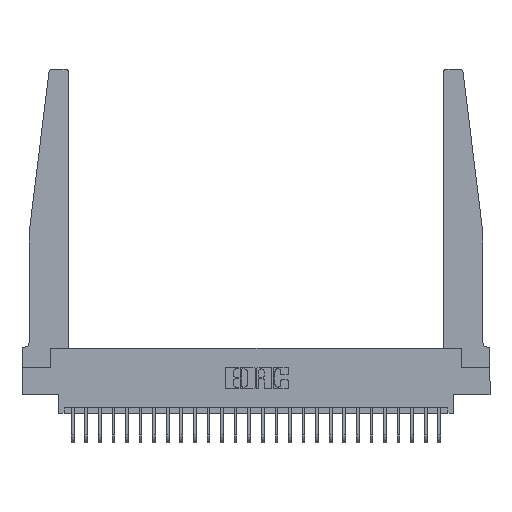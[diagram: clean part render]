
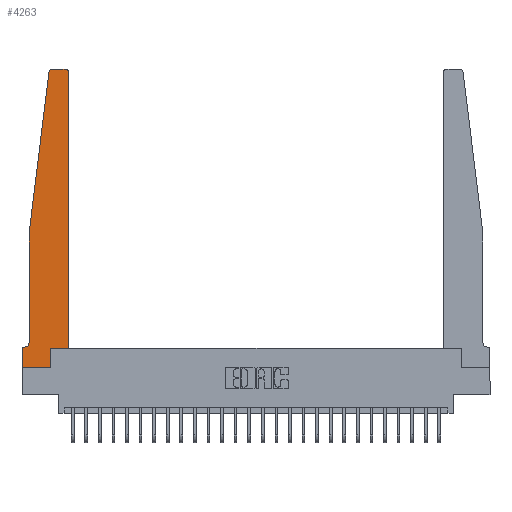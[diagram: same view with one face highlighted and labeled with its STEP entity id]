
A CAD part, top view. The second image highlights one B-rep face of the part: STEP entity #4263.
In plain terms, the highlighted planar face has unit normal (0, 0, 1).
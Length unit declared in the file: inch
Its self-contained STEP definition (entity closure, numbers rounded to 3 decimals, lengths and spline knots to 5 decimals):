
#93 = CARTESIAN_POINT ( 'NONE',  ( 0.425, 0.18, 0.37 ) ) ;
#144 = CARTESIAN_POINT ( 'NONE',  ( 0.015, 0.1875, 0.37 ) ) ;
#381 = DIRECTION ( 'NONE',  ( 1., 0., 0. ) ) ;
#610 = VECTOR ( 'NONE', #15739, 39.37008 ) ;
#1240 = AXIS2_PLACEMENT_3D ( 'NONE', #2203, #24949, #12525 ) ;
#1258 = CARTESIAN_POINT ( 'NONE',  ( 0.065, 0.1875, 0.37 ) ) ;
#2203 = CARTESIAN_POINT ( 'NONE',  ( 0.27653, 2.72, 0.37 ) ) ;
#2402 = CARTESIAN_POINT ( 'NONE',  ( 0.425, 0.18, 0.37 ) ) ;
#2494 = CARTESIAN_POINT ( 'NONE',  ( 0.2605, 0.18, 0.37 ) ) ;
#3144 = LINE ( 'NONE', #6841, #13518 ) ;
#3421 = ORIENTED_EDGE ( 'NONE', *, *, #20237, .T. ) ;
#3895 = LINE ( 'NONE', #1258, #610 ) ;
#4263 = ADVANCED_FACE ( 'NONE', ( #12003 ), #23340, .T. ) ;
#4941 = EDGE_CURVE ( 'NONE', #6797, #12315, #3895, .T. ) ;
#4987 = ORIENTED_EDGE ( 'NONE', *, *, #25589, .T. ) ;
#5059 = VERTEX_POINT ( 'NONE', #24735 ) ;
#5193 = CARTESIAN_POINT ( 'NONE',  ( 0.015, 0.2375, 0.37 ) ) ;
#5317 = EDGE_CURVE ( 'NONE', #20137, #15639, #16527, .T. ) ;
#5744 = CARTESIAN_POINT ( 'NONE',  ( 0., 0., 0.37 ) ) ;
#6098 = ORIENTED_EDGE ( 'NONE', *, *, #21970, .T. ) ;
#6454 = LINE ( 'NONE', #19128, #8363 ) ;
#6511 = LINE ( 'NONE', #9310, #22659 ) ;
#6797 = VERTEX_POINT ( 'NONE', #144 ) ;
#6841 = CARTESIAN_POINT ( 'NONE',  ( 0.25, 2.75, 0.37 ) ) ;
#7742 = EDGE_CURVE ( 'NONE', #5059, #6797, #14468, .T. ) ;
#7963 = ORIENTED_EDGE ( 'NONE', *, *, #19865, .T. ) ;
#8076 = DIRECTION ( 'NONE',  ( 1., 0., 0. ) ) ;
#8299 = CARTESIAN_POINT ( 'NONE',  ( 0.27653, 2.75, 0.37 ) ) ;
#8310 = AXIS2_PLACEMENT_3D ( 'NONE', #5193, #21519, #15535 ) ;
#8363 = VECTOR ( 'NONE', #10907, 39.37008 ) ;
#8761 = AXIS2_PLACEMENT_3D ( 'NONE', #12805, #14875, #381 ) ;
#8945 = EDGE_CURVE ( 'NONE', #13265, #20823, #6454, .T. ) ;
#9310 = CARTESIAN_POINT ( 'NONE',  ( 0., 0., 0.37 ) ) ;
#9668 = VERTEX_POINT ( 'NONE', #93 ) ;
#9821 = ORIENTED_EDGE ( 'NONE', *, *, #10875, .T. ) ;
#10350 = VECTOR ( 'NONE', #23063, 39.37008 ) ;
#10642 = CARTESIAN_POINT ( 'NONE',  ( 0.065, 1.25, 0.37 ) ) ;
#10706 = VERTEX_POINT ( 'NONE', #22304 ) ;
#10799 = VECTOR ( 'NONE', #16868, 39.37008 ) ;
#10838 = DIRECTION ( 'NONE',  ( 1., 0., 0. ) ) ;
#10875 = EDGE_CURVE ( 'NONE', #20823, #5059, #24450, .T. ) ;
#10907 = DIRECTION ( 'NONE',  ( -0.122, -0.992, 0. ) ) ;
#12003 = FACE_OUTER_BOUND ( 'NONE', #17654, .T. ) ;
#12041 = ORIENTED_EDGE ( 'NONE', *, *, #14633, .T. ) ;
#12166 = ORIENTED_EDGE ( 'NONE', *, *, #8945, .T. ) ;
#12193 = DIRECTION ( 'NONE',  ( 1., 0., 0. ) ) ;
#12315 = VERTEX_POINT ( 'NONE', #18004 ) ;
#12525 = DIRECTION ( 'NONE',  ( 1., 0., 0. ) ) ;
#12805 = CARTESIAN_POINT ( 'NONE',  ( 0.395, 2.72, 0.37 ) ) ;
#13265 = VERTEX_POINT ( 'NONE', #14531 ) ;
#13296 = VECTOR ( 'NONE', #12193, 39.37008 ) ;
#13518 = VECTOR ( 'NONE', #21376, 39.37008 ) ;
#13732 = CARTESIAN_POINT ( 'NONE',  ( 0.2605, 0., 0.37 ) ) ;
#14061 = EDGE_CURVE ( 'NONE', #15639, #21024, #18441, .T. ) ;
#14216 = CARTESIAN_POINT ( 'NONE',  ( 0.425, 0.18, 0.37 ) ) ;
#14468 = CIRCLE ( 'NONE', #8310, 0.05 ) ;
#14531 = CARTESIAN_POINT ( 'NONE',  ( 0.24675, 2.72367, 0.37 ) ) ;
#14633 = EDGE_CURVE ( 'NONE', #12315, #20137, #6511, .T. ) ;
#14875 = DIRECTION ( 'NONE',  ( 0., 0., 1. ) ) ;
#15185 = CIRCLE ( 'NONE', #1240, 0.03 ) ;
#15229 = CIRCLE ( 'NONE', #8761, 0.03 ) ;
#15535 = DIRECTION ( 'NONE',  ( -1., 0., 0. ) ) ;
#15639 = VERTEX_POINT ( 'NONE', #13732 ) ;
#15739 = DIRECTION ( 'NONE',  ( -1., 0., 0. ) ) ;
#16478 = AXIS2_PLACEMENT_3D ( 'NONE', #16970, #17331, #10838 ) ;
#16527 = LINE ( 'NONE', #5744, #13296 ) ;
#16868 = DIRECTION ( 'NONE',  ( 0., 1., 0. ) ) ;
#16948 = ORIENTED_EDGE ( 'NONE', *, *, #14061, .T. ) ;
#16970 = CARTESIAN_POINT ( 'NONE',  ( 0., 0.1875, 0.37 ) ) ;
#17062 = CARTESIAN_POINT ( 'NONE',  ( 0., 0., 0.37 ) ) ;
#17125 = EDGE_CURVE ( 'NONE', #21081, #21837, #3144, .T. ) ;
#17331 = DIRECTION ( 'NONE',  ( 0., 0., 1. ) ) ;
#17654 = EDGE_LOOP ( 'NONE', ( #20307, #4987, #12166, #9821, #26790, #18220, #12041, #24523, #16948, #7963, #3421, #6098 ) ) ;
#17679 = CARTESIAN_POINT ( 'NONE',  ( 0.395, 2.75, 0.37 ) ) ;
#17789 = DIRECTION ( 'NONE',  ( 0., -1., 0. ) ) ;
#18004 = CARTESIAN_POINT ( 'NONE',  ( 0., 0.1875, 0.37 ) ) ;
#18220 = ORIENTED_EDGE ( 'NONE', *, *, #4941, .T. ) ;
#18441 = LINE ( 'NONE', #2494, #10350 ) ;
#18624 = CARTESIAN_POINT ( 'NONE',  ( 0.065, 1.25, 0.37 ) ) ;
#19128 = CARTESIAN_POINT ( 'NONE',  ( 0.065, 1.25, 0.37 ) ) ;
#19861 = LINE ( 'NONE', #14216, #25419 ) ;
#19865 = EDGE_CURVE ( 'NONE', #21024, #9668, #19861, .T. ) ;
#20137 = VERTEX_POINT ( 'NONE', #17062 ) ;
#20237 = EDGE_CURVE ( 'NONE', #9668, #10706, #23435, .T. ) ;
#20307 = ORIENTED_EDGE ( 'NONE', *, *, #17125, .T. ) ;
#20823 = VERTEX_POINT ( 'NONE', #18624 ) ;
#21024 = VERTEX_POINT ( 'NONE', #23963 ) ;
#21081 = VERTEX_POINT ( 'NONE', #17679 ) ;
#21376 = DIRECTION ( 'NONE',  ( -1., 0., 0. ) ) ;
#21519 = DIRECTION ( 'NONE',  ( 0., 0., -1. ) ) ;
#21837 = VERTEX_POINT ( 'NONE', #8299 ) ;
#21970 = EDGE_CURVE ( 'NONE', #10706, #21081, #15229, .T. ) ;
#22304 = CARTESIAN_POINT ( 'NONE',  ( 0.425, 2.72, 0.37 ) ) ;
#22659 = VECTOR ( 'NONE', #17789, 39.37008 ) ;
#23063 = DIRECTION ( 'NONE',  ( 0., 1., 0. ) ) ;
#23340 = PLANE ( 'NONE',  #16478 ) ;
#23435 = LINE ( 'NONE', #2402, #10799 ) ;
#23963 = CARTESIAN_POINT ( 'NONE',  ( 0.2605, 0.18, 0.37 ) ) ;
#24114 = VECTOR ( 'NONE', #26814, 39.37008 ) ;
#24450 = LINE ( 'NONE', #10642, #24114 ) ;
#24523 = ORIENTED_EDGE ( 'NONE', *, *, #5317, .T. ) ;
#24735 = CARTESIAN_POINT ( 'NONE',  ( 0.065, 0.2375, 0.37 ) ) ;
#24949 = DIRECTION ( 'NONE',  ( 0., 0., 1. ) ) ;
#25419 = VECTOR ( 'NONE', #8076, 39.37008 ) ;
#25589 = EDGE_CURVE ( 'NONE', #21837, #13265, #15185, .T. ) ;
#26790 = ORIENTED_EDGE ( 'NONE', *, *, #7742, .T. ) ;
#26814 = DIRECTION ( 'NONE',  ( 0., -1., 0. ) ) ;
